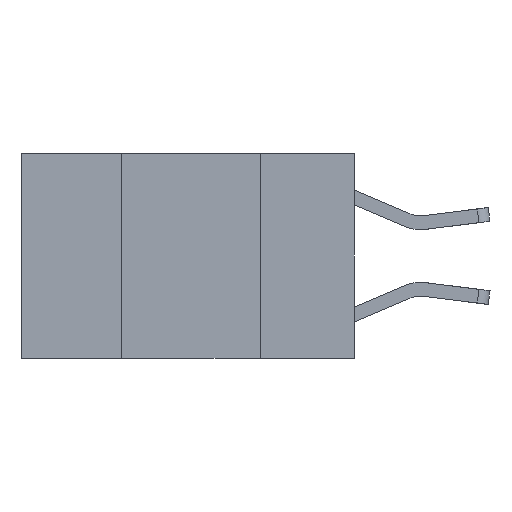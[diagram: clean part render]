
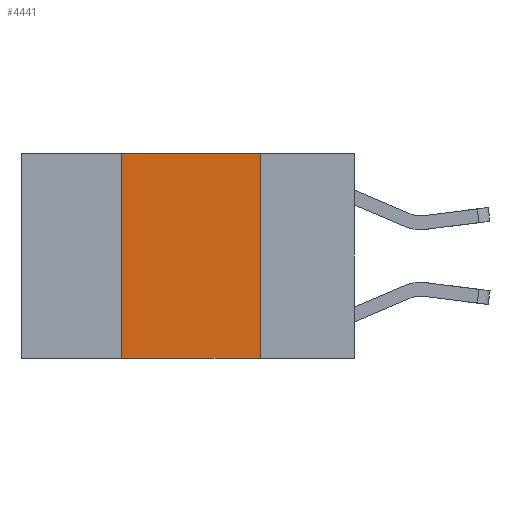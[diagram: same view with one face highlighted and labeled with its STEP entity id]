
A CAD part, left-side view. The second image highlights one B-rep face of the part: STEP entity #4441.
In plain terms, the highlighted planar face has unit normal (-1, 0, 0).
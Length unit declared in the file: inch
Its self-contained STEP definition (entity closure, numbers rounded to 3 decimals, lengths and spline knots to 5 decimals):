
#4 = CARTESIAN_POINT ( 'NONE',  ( 0., 0.17, 0. ) ) ;
#111 = CARTESIAN_POINT ( 'NONE',  ( 0., 0.6, 0. ) ) ;
#440 = EDGE_LOOP ( 'NONE', ( #9167, #6524, #9581, #9463 ) ) ;
#590 = VECTOR ( 'NONE', #7109, 39.37008 ) ;
#1086 = PLANE ( 'NONE',  #2558 ) ;
#1131 = LINE ( 'NONE', #9398, #10556 ) ;
#1646 = VECTOR ( 'NONE', #9988, 39.37008 ) ;
#2558 = AXIS2_PLACEMENT_3D ( 'NONE', #111, #8524, #2985 ) ;
#2826 = LINE ( 'NONE', #3018, #590 ) ;
#2985 = DIRECTION ( 'NONE',  ( 0., 0., -1. ) ) ;
#3018 = CARTESIAN_POINT ( 'NONE',  ( 0., 0.17, 0. ) ) ;
#3486 = VERTEX_POINT ( 'NONE', #6525 ) ;
#3629 = EDGE_CURVE ( 'NONE', #11277, #4344, #2826, .T. ) ;
#4047 = EDGE_CURVE ( 'NONE', #5986, #4344, #8728, .T. ) ;
#4344 = VERTEX_POINT ( 'NONE', #8252 ) ;
#4441 = ADVANCED_FACE ( 'NONE', ( #9112 ), #1086, .F. ) ;
#4900 = EDGE_CURVE ( 'NONE', #3486, #11277, #9516, .T. ) ;
#5519 = CARTESIAN_POINT ( 'NONE',  ( 0., 0.6, -0.37 ) ) ;
#5570 = CARTESIAN_POINT ( 'NONE',  ( 0., 0.42, -0.37 ) ) ;
#5986 = VERTEX_POINT ( 'NONE', #5570 ) ;
#6524 = ORIENTED_EDGE ( 'NONE', *, *, #4900, .F. ) ;
#6525 = CARTESIAN_POINT ( 'NONE',  ( 0., 0.42, 0. ) ) ;
#7109 = DIRECTION ( 'NONE',  ( 0., 0., -1. ) ) ;
#7136 = CARTESIAN_POINT ( 'NONE',  ( 0., 0.6, 0. ) ) ;
#7698 = EDGE_CURVE ( 'NONE', #5986, #3486, #1131, .T. ) ;
#8252 = CARTESIAN_POINT ( 'NONE',  ( 0., 0.17, -0.37 ) ) ;
#8524 = DIRECTION ( 'NONE',  ( 1., 0., 0. ) ) ;
#8526 = DIRECTION ( 'NONE',  ( 0., 0., 1. ) ) ;
#8728 = LINE ( 'NONE', #5519, #1646 ) ;
#9112 = FACE_OUTER_BOUND ( 'NONE', #440, .T. ) ;
#9167 = ORIENTED_EDGE ( 'NONE', *, *, #3629, .F. ) ;
#9398 = CARTESIAN_POINT ( 'NONE',  ( 0., 0.42, 0. ) ) ;
#9463 = ORIENTED_EDGE ( 'NONE', *, *, #4047, .T. ) ;
#9516 = LINE ( 'NONE', #7136, #11542 ) ;
#9581 = ORIENTED_EDGE ( 'NONE', *, *, #7698, .F. ) ;
#9988 = DIRECTION ( 'NONE',  ( 0., -1., 0. ) ) ;
#10528 = DIRECTION ( 'NONE',  ( 0., -1., 0. ) ) ;
#10556 = VECTOR ( 'NONE', #8526, 39.37008 ) ;
#11277 = VERTEX_POINT ( 'NONE', #4 ) ;
#11542 = VECTOR ( 'NONE', #10528, 39.37008 ) ;
